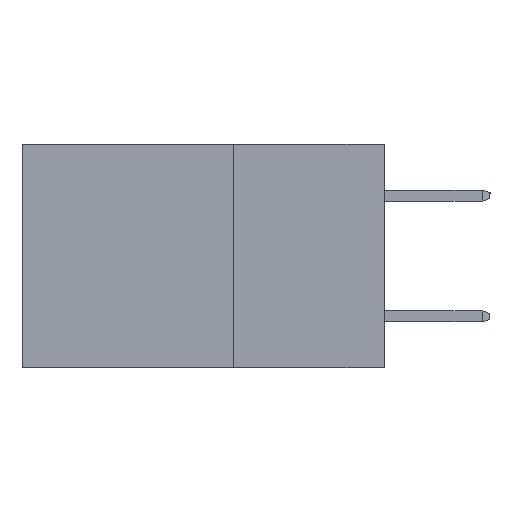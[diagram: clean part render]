
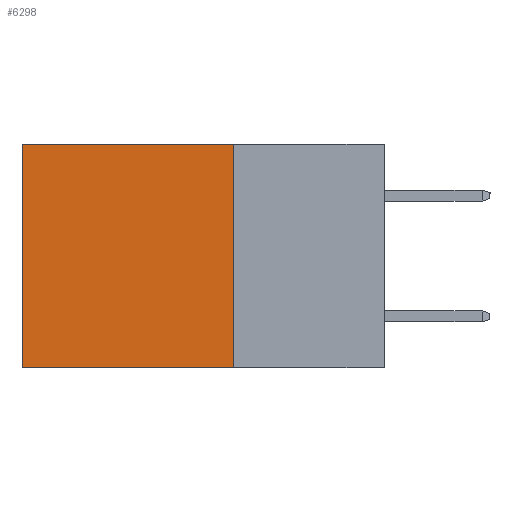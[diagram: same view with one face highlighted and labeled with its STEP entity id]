
A CAD part, left-side view. The second image highlights one B-rep face of the part: STEP entity #6298.
In plain terms, the highlighted planar face has unit normal (-1, 0, 0).
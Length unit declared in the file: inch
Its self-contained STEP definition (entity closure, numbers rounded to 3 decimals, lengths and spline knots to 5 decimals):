
#35 = VECTOR ( 'NONE', #8370, 39.37008 ) ;
#154 = CARTESIAN_POINT ( 'NONE',  ( 0.2615, 0.6, -0.37 ) ) ;
#605 = CARTESIAN_POINT ( 'NONE',  ( 0.2615, 0.25, -0.37 ) ) ;
#613 = ORIENTED_EDGE ( 'NONE', *, *, #5010, .T. ) ;
#1746 = VERTEX_POINT ( 'NONE', #5092 ) ;
#2071 = VECTOR ( 'NONE', #4876, 39.37008 ) ;
#2233 = VECTOR ( 'NONE', #6748, 39.37008 ) ;
#2970 = AXIS2_PLACEMENT_3D ( 'NONE', #13920, #5841, #5918 ) ;
#3136 = EDGE_LOOP ( 'NONE', ( #613, #9379, #7682, #7796 ) ) ;
#3228 = EDGE_CURVE ( 'NONE', #3416, #13232, #13844, .T. ) ;
#3416 = VERTEX_POINT ( 'NONE', #8827 ) ;
#3443 = LINE ( 'NONE', #8278, #14725 ) ;
#3606 = EDGE_CURVE ( 'NONE', #13232, #1746, #3443, .T. ) ;
#4507 = FACE_OUTER_BOUND ( 'NONE', #3136, .T. ) ;
#4876 = DIRECTION ( 'NONE',  ( 0., 1., 0. ) ) ;
#5010 = EDGE_CURVE ( 'NONE', #10608, #1746, #6965, .T. ) ;
#5092 = CARTESIAN_POINT ( 'NONE',  ( 0.2615, 0.6, -0.37 ) ) ;
#5243 = EDGE_CURVE ( 'NONE', #3416, #10608, #5991, .T. ) ;
#5841 = DIRECTION ( 'NONE',  ( 1., 0., 0. ) ) ;
#5918 = DIRECTION ( 'NONE',  ( 0., 0., -1. ) ) ;
#5991 = LINE ( 'NONE', #10534, #2071 ) ;
#6298 = ADVANCED_FACE ( 'NONE', ( #4507 ), #9065, .F. ) ;
#6748 = DIRECTION ( 'NONE',  ( 0., 0., -1. ) ) ;
#6965 = LINE ( 'NONE', #154, #2233 ) ;
#7682 = ORIENTED_EDGE ( 'NONE', *, *, #3228, .F. ) ;
#7796 = ORIENTED_EDGE ( 'NONE', *, *, #5243, .T. ) ;
#8278 = CARTESIAN_POINT ( 'NONE',  ( 0.2615, 0.25, -0.37 ) ) ;
#8370 = DIRECTION ( 'NONE',  ( 0., 0., -1. ) ) ;
#8827 = CARTESIAN_POINT ( 'NONE',  ( 0.2615, 0.25, 0. ) ) ;
#8848 = CARTESIAN_POINT ( 'NONE',  ( 0.2615, 0.6, 0. ) ) ;
#9065 = PLANE ( 'NONE',  #2970 ) ;
#9379 = ORIENTED_EDGE ( 'NONE', *, *, #3606, .F. ) ;
#9404 = DIRECTION ( 'NONE',  ( 0., 1., 0. ) ) ;
#10534 = CARTESIAN_POINT ( 'NONE',  ( 0.2615, 0.25, 0. ) ) ;
#10608 = VERTEX_POINT ( 'NONE', #8848 ) ;
#11678 = CARTESIAN_POINT ( 'NONE',  ( 0.2615, 0.25, -0.37 ) ) ;
#13232 = VERTEX_POINT ( 'NONE', #605 ) ;
#13844 = LINE ( 'NONE', #11678, #35 ) ;
#13920 = CARTESIAN_POINT ( 'NONE',  ( 0.2615, 0.25, -0.37 ) ) ;
#14725 = VECTOR ( 'NONE', #9404, 39.37008 ) ;
